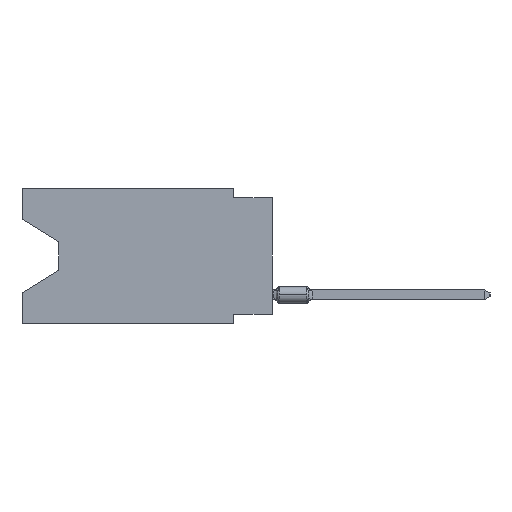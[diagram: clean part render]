
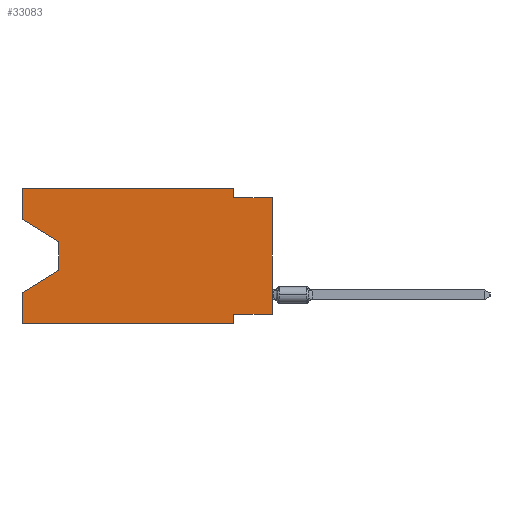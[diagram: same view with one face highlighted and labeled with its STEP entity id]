
A CAD part, left-side view. The second image highlights one B-rep face of the part: STEP entity #33083.
In plain terms, the highlighted planar face has unit normal (-1, 0, 0).
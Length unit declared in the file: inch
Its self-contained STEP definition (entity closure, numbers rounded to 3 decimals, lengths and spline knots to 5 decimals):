
#497 = VERTEX_POINT ( 'NONE', #20754 ) ;
#1156 = EDGE_CURVE ( 'NONE', #20580, #30942, #12106, .T. ) ;
#1507 = CARTESIAN_POINT ( 'NONE',  ( 0., 0.1, -0.35 ) ) ;
#1664 = VECTOR ( 'NONE', #5727, 39.37008 ) ;
#1997 = VECTOR ( 'NONE', #24584, 39.37008 ) ;
#2043 = DIRECTION ( 'NONE',  ( 0., 0., -1. ) ) ;
#2282 = VERTEX_POINT ( 'NONE', #4337 ) ;
#2326 = LINE ( 'NONE', #9981, #25398 ) ;
#2957 = VECTOR ( 'NONE', #3482, 39.37008 ) ;
#3399 = CARTESIAN_POINT ( 'NONE',  ( 0., 0., -0.325 ) ) ;
#3482 = DIRECTION ( 'NONE',  ( 0., -1., 0. ) ) ;
#3494 = CARTESIAN_POINT ( 'NONE',  ( 0., 0.645, -0.08025 ) ) ;
#3676 = EDGE_CURVE ( 'NONE', #31476, #29472, #27743, .T. ) ;
#3746 = DIRECTION ( 'NONE',  ( 0., 0., 1. ) ) ;
#4337 = CARTESIAN_POINT ( 'NONE',  ( 0., 0.55, -0.138 ) ) ;
#4736 = EDGE_CURVE ( 'NONE', #13287, #16098, #32751, .T. ) ;
#4925 = VECTOR ( 'NONE', #25159, 39.37008 ) ;
#5090 = CARTESIAN_POINT ( 'NONE',  ( 0., 0., -0.025 ) ) ;
#5727 = DIRECTION ( 'NONE',  ( 0., 0., -1. ) ) ;
#6229 = VECTOR ( 'NONE', #14247, 39.37008 ) ;
#6504 = CARTESIAN_POINT ( 'NONE',  ( 0., 0.645, 0. ) ) ;
#6584 = CARTESIAN_POINT ( 'NONE',  ( 0., 0.645, -0.35 ) ) ;
#7428 = CARTESIAN_POINT ( 'NONE',  ( 0., 0.645, -0.08025 ) ) ;
#7883 = EDGE_CURVE ( 'NONE', #20580, #2282, #20932, .T. ) ;
#7893 = CARTESIAN_POINT ( 'NONE',  ( 0., 0.1, 0. ) ) ;
#8071 = CARTESIAN_POINT ( 'NONE',  ( 0., 0.1, -0.025 ) ) ;
#8449 = CARTESIAN_POINT ( 'NONE',  ( 0., 0.645, 0. ) ) ;
#8846 = EDGE_CURVE ( 'NONE', #2282, #24016, #19479, .T. ) ;
#9330 = AXIS2_PLACEMENT_3D ( 'NONE', #8449, #21425, #16262 ) ;
#9835 = EDGE_CURVE ( 'NONE', #24016, #14899, #18575, .T. ) ;
#9981 = CARTESIAN_POINT ( 'NONE',  ( 0., 0.645, 0. ) ) ;
#10096 = VECTOR ( 'NONE', #2043, 39.37008 ) ;
#10239 = CARTESIAN_POINT ( 'NONE',  ( 0., 0.1, -0.325 ) ) ;
#10625 = VECTOR ( 'NONE', #15380, 39.37008 ) ;
#10762 = FACE_OUTER_BOUND ( 'NONE', #21020, .T. ) ;
#11087 = LINE ( 'NONE', #16239, #1997 ) ;
#11152 = LINE ( 'NONE', #6504, #2957 ) ;
#11457 = ORIENTED_EDGE ( 'NONE', *, *, #12975, .T. ) ;
#12040 = VECTOR ( 'NONE', #26429, 39.37008 ) ;
#12106 = LINE ( 'NONE', #25081, #14189 ) ;
#12272 = VECTOR ( 'NONE', #33156, 39.37008 ) ;
#12975 = EDGE_CURVE ( 'NONE', #33758, #20077, #11087, .T. ) ;
#13287 = VERTEX_POINT ( 'NONE', #17803 ) ;
#13765 = EDGE_CURVE ( 'NONE', #16098, #497, #18250, .T. ) ;
#14099 = EDGE_CURVE ( 'NONE', #29472, #20077, #15724, .T. ) ;
#14189 = VECTOR ( 'NONE', #3746, 39.37008 ) ;
#14247 = DIRECTION ( 'NONE',  ( 0., 1., 0. ) ) ;
#14331 = ORIENTED_EDGE ( 'NONE', *, *, #4736, .F. ) ;
#14899 = VERTEX_POINT ( 'NONE', #27363 ) ;
#15380 = DIRECTION ( 'NONE',  ( 0., 0.855, -0.519 ) ) ;
#15724 = LINE ( 'NONE', #1507, #10096 ) ;
#16098 = VERTEX_POINT ( 'NONE', #8071 ) ;
#16239 = CARTESIAN_POINT ( 'NONE',  ( 0., 0.645, -0.35 ) ) ;
#16262 = DIRECTION ( 'NONE',  ( 0., 0., -1. ) ) ;
#16991 = CARTESIAN_POINT ( 'NONE',  ( 0., 0.55, -0.138 ) ) ;
#17649 = EDGE_CURVE ( 'NONE', #33758, #14899, #2326, .T. ) ;
#17803 = CARTESIAN_POINT ( 'NONE',  ( 0., 0.1, 0. ) ) ;
#18250 = LINE ( 'NONE', #5090, #25948 ) ;
#18575 = LINE ( 'NONE', #21058, #10625 ) ;
#19033 = ORIENTED_EDGE ( 'NONE', *, *, #8846, .T. ) ;
#19130 = LINE ( 'NONE', #22303, #12272 ) ;
#19479 = LINE ( 'NONE', #16991, #4925 ) ;
#20077 = VERTEX_POINT ( 'NONE', #22557 ) ;
#20580 = VERTEX_POINT ( 'NONE', #3494 ) ;
#20754 = CARTESIAN_POINT ( 'NONE',  ( 0., 0., -0.025 ) ) ;
#20760 = ORIENTED_EDGE ( 'NONE', *, *, #3676, .F. ) ;
#20824 = ORIENTED_EDGE ( 'NONE', *, *, #35037, .T. ) ;
#20932 = LINE ( 'NONE', #7428, #12040 ) ;
#21020 = EDGE_LOOP ( 'NONE', ( #31676, #19033, #31507, #27631, #11457, #34002, #20760, #20824, #31873, #14331, #29026, #32741 ) ) ;
#21058 = CARTESIAN_POINT ( 'NONE',  ( 0., 0.55, -0.212 ) ) ;
#21425 = DIRECTION ( 'NONE',  ( 1., 0., 0. ) ) ;
#22303 = CARTESIAN_POINT ( 'NONE',  ( 0., 0., 0. ) ) ;
#22557 = CARTESIAN_POINT ( 'NONE',  ( 0., 0.1, -0.35 ) ) ;
#23401 = DIRECTION ( 'NONE',  ( 0., -1., 0. ) ) ;
#23973 = CARTESIAN_POINT ( 'NONE',  ( 0., 0.645, 0. ) ) ;
#24016 = VERTEX_POINT ( 'NONE', #33343 ) ;
#24584 = DIRECTION ( 'NONE',  ( 0., -1., 0. ) ) ;
#25081 = CARTESIAN_POINT ( 'NONE',  ( 0., 0.645, 0. ) ) ;
#25159 = DIRECTION ( 'NONE',  ( 0., 0., -1. ) ) ;
#25398 = VECTOR ( 'NONE', #32009, 39.37008 ) ;
#25948 = VECTOR ( 'NONE', #23401, 39.37008 ) ;
#26429 = DIRECTION ( 'NONE',  ( 0., -0.855, -0.519 ) ) ;
#27363 = CARTESIAN_POINT ( 'NONE',  ( 0., 0.645, -0.26975 ) ) ;
#27631 = ORIENTED_EDGE ( 'NONE', *, *, #17649, .F. ) ;
#27743 = LINE ( 'NONE', #3399, #6229 ) ;
#28012 = EDGE_CURVE ( 'NONE', #30942, #13287, #11152, .T. ) ;
#29026 = ORIENTED_EDGE ( 'NONE', *, *, #28012, .F. ) ;
#29472 = VERTEX_POINT ( 'NONE', #10239 ) ;
#30942 = VERTEX_POINT ( 'NONE', #23973 ) ;
#31476 = VERTEX_POINT ( 'NONE', #32987 ) ;
#31507 = ORIENTED_EDGE ( 'NONE', *, *, #9835, .T. ) ;
#31676 = ORIENTED_EDGE ( 'NONE', *, *, #7883, .T. ) ;
#31873 = ORIENTED_EDGE ( 'NONE', *, *, #13765, .F. ) ;
#32009 = DIRECTION ( 'NONE',  ( 0., 0., 1. ) ) ;
#32264 = PLANE ( 'NONE',  #9330 ) ;
#32741 = ORIENTED_EDGE ( 'NONE', *, *, #1156, .F. ) ;
#32751 = LINE ( 'NONE', #7893, #1664 ) ;
#32987 = CARTESIAN_POINT ( 'NONE',  ( 0., 0., -0.325 ) ) ;
#33083 = ADVANCED_FACE ( 'NONE', ( #10762 ), #32264, .F. ) ;
#33156 = DIRECTION ( 'NONE',  ( 0., 0., 1. ) ) ;
#33343 = CARTESIAN_POINT ( 'NONE',  ( 0., 0.55, -0.212 ) ) ;
#33758 = VERTEX_POINT ( 'NONE', #6584 ) ;
#34002 = ORIENTED_EDGE ( 'NONE', *, *, #14099, .F. ) ;
#35037 = EDGE_CURVE ( 'NONE', #31476, #497, #19130, .T. ) ;
